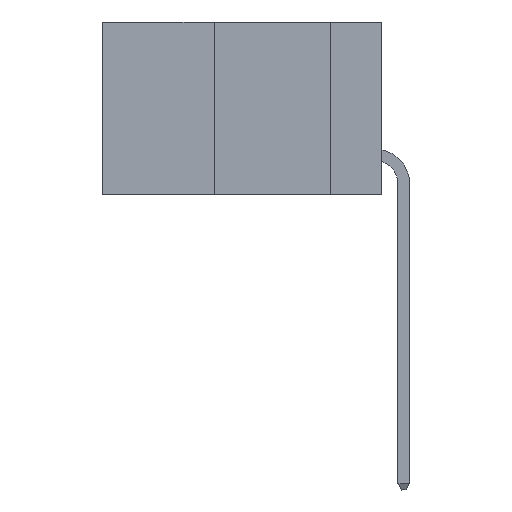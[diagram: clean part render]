
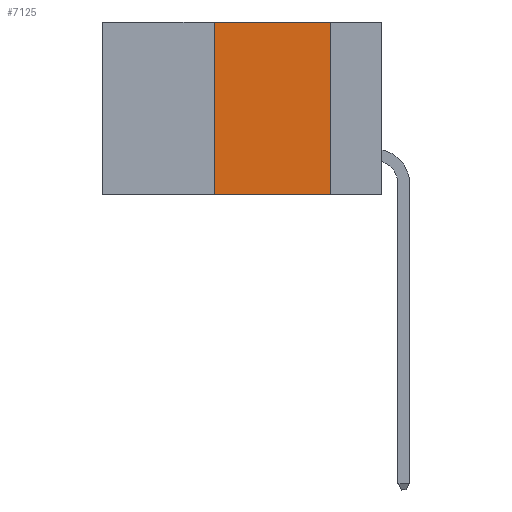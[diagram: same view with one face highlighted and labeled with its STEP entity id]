
A CAD part, left-side view. The second image highlights one B-rep face of the part: STEP entity #7125.
In plain terms, the highlighted planar face has unit normal (-1, 0, 0).
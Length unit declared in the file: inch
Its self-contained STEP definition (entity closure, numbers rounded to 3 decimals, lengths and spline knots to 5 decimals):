
#314 = CARTESIAN_POINT ( 'NONE',  ( 0., 0.36, 0. ) ) ;
#356 = PLANE ( 'NONE',  #2962 ) ;
#411 = DIRECTION ( 'NONE',  ( 0., 0., -1. ) ) ;
#885 = CARTESIAN_POINT ( 'NONE',  ( 0., 0.6, 0. ) ) ;
#1136 = VERTEX_POINT ( 'NONE', #14894 ) ;
#1267 = ORIENTED_EDGE ( 'NONE', *, *, #9833, .T. ) ;
#1522 = EDGE_CURVE ( 'NONE', #9204, #10763, #9557, .T. ) ;
#1551 = CARTESIAN_POINT ( 'NONE',  ( 0., 0.6, 0. ) ) ;
#2859 = VECTOR ( 'NONE', #12179, 39.37008 ) ;
#2962 = AXIS2_PLACEMENT_3D ( 'NONE', #1551, #14303, #411 ) ;
#3177 = DIRECTION ( 'NONE',  ( 0., 0., -1. ) ) ;
#3458 = DIRECTION ( 'NONE',  ( 0., 0., 1. ) ) ;
#3753 = LINE ( 'NONE', #7908, #3950 ) ;
#3950 = VECTOR ( 'NONE', #3177, 39.37008 ) ;
#3996 = CARTESIAN_POINT ( 'NONE',  ( 0., 0.6, -0.37 ) ) ;
#4470 = DIRECTION ( 'NONE',  ( 0., -1., 0. ) ) ;
#5272 = ORIENTED_EDGE ( 'NONE', *, *, #5979, .F. ) ;
#5544 = CARTESIAN_POINT ( 'NONE',  ( 0., 0.11, 0. ) ) ;
#5979 = EDGE_CURVE ( 'NONE', #7736, #9204, #13994, .T. ) ;
#6181 = VECTOR ( 'NONE', #3458, 39.37008 ) ;
#7125 = ADVANCED_FACE ( 'NONE', ( #12706 ), #356, .F. ) ;
#7736 = VERTEX_POINT ( 'NONE', #11001 ) ;
#7908 = CARTESIAN_POINT ( 'NONE',  ( 0., 0.11, 0. ) ) ;
#9204 = VERTEX_POINT ( 'NONE', #314 ) ;
#9305 = EDGE_LOOP ( 'NONE', ( #9935, #10886, #5272, #1267 ) ) ;
#9557 = LINE ( 'NONE', #885, #13362 ) ;
#9833 = EDGE_CURVE ( 'NONE', #7736, #1136, #11648, .T. ) ;
#9935 = ORIENTED_EDGE ( 'NONE', *, *, #10025, .F. ) ;
#10025 = EDGE_CURVE ( 'NONE', #10763, #1136, #3753, .T. ) ;
#10763 = VERTEX_POINT ( 'NONE', #5544 ) ;
#10886 = ORIENTED_EDGE ( 'NONE', *, *, #1522, .F. ) ;
#11001 = CARTESIAN_POINT ( 'NONE',  ( 0., 0.36, -0.37 ) ) ;
#11648 = LINE ( 'NONE', #3996, #2859 ) ;
#11737 = CARTESIAN_POINT ( 'NONE',  ( 0., 0.36, 0. ) ) ;
#12179 = DIRECTION ( 'NONE',  ( 0., -1., 0. ) ) ;
#12706 = FACE_OUTER_BOUND ( 'NONE', #9305, .T. ) ;
#13362 = VECTOR ( 'NONE', #4470, 39.37008 ) ;
#13994 = LINE ( 'NONE', #11737, #6181 ) ;
#14303 = DIRECTION ( 'NONE',  ( 1., 0., 0. ) ) ;
#14894 = CARTESIAN_POINT ( 'NONE',  ( 0., 0.11, -0.37 ) ) ;
